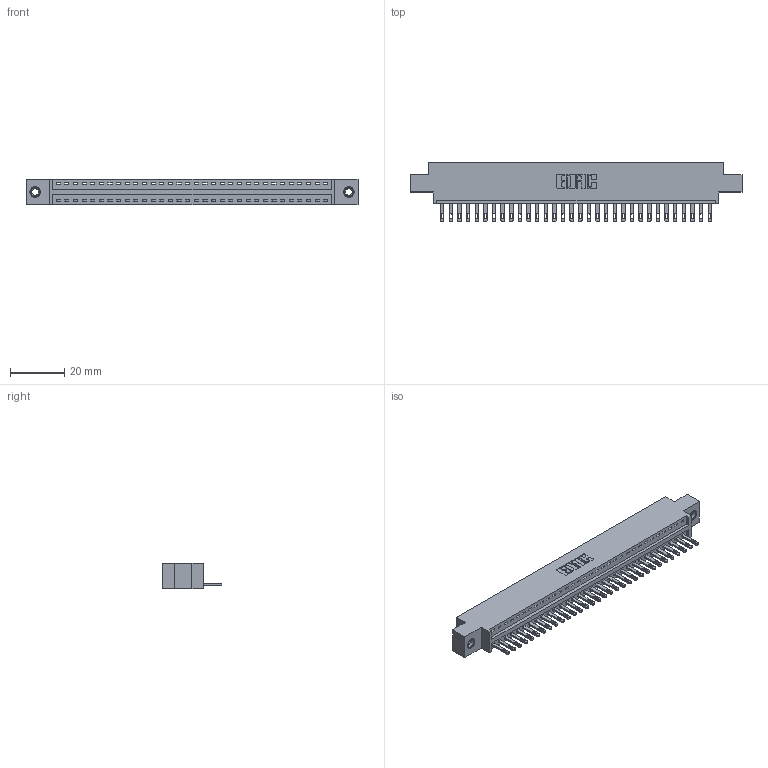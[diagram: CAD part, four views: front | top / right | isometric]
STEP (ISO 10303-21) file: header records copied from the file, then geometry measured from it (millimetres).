
FILE_DESCRIPTION (( 'STEP AP203' ), '1' );
FILE_NAME ('346-032-500-607.STEP', '2018-08-22T07:50:39', ( '' ), ( '' ), 'SwSTEP 2.0', 'SolidWorks 2016', '' );
FILE_SCHEMA (( 'CONFIG_CONTROL_DESIGN' ));
Length unit declared in the file: inch
Products named in the file (4): 345-292-001_345-293-100; 345-250-001_345-250-005-103; 346-032-500-607; 346 Part_0.170 Offset - 0.156 Dia-TI
Assembly tree (35 placements, depth 2):
  346-032-500-607
    346 Part_0.170 Offset - 0.156 Dia-TI
    345-292-001_345-293-100  x32
    345-250-001_345-250-005-103  x2
Bounding box: 122.17 x 21.84 x 9.4 mm (x, y, z)
Volume: 11477.5 mm3; surface area: 14507.1 mm2
Topology: 35 solids, 35 shells, 1914 faces, 5853 edges, 3894 vertices
Faces by surface type: plane 1200, cylinder 698, cone 12, torus 4
Entity records: 22454 total; most frequent: CARTESIAN_POINT 3835, ORIENTED_EDGE 3794, DIRECTION 3423, EDGE_CURVE 1897, VECTOR 1613, LINE 1613, VERTEX_POINT 1260, AXIS2_PLACEMENT_3D 905
